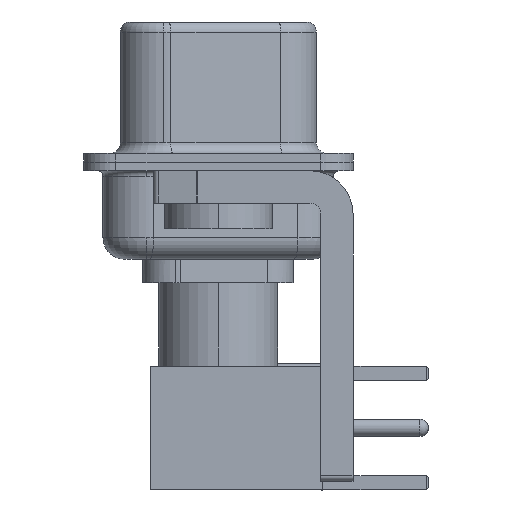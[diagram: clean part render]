
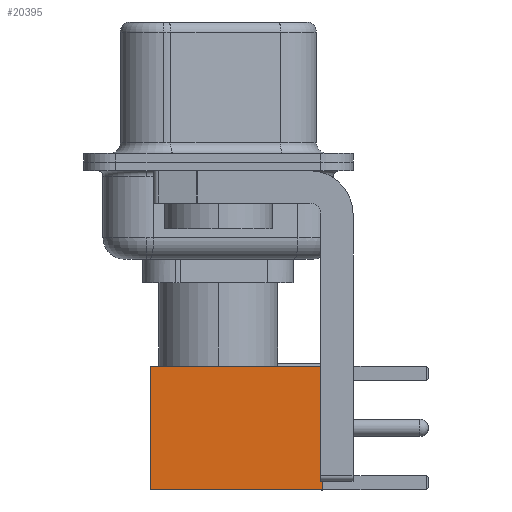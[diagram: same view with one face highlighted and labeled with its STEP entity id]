
A CAD part, left-side view. The second image highlights one B-rep face of the part: STEP entity #20395.
In plain terms, the highlighted face is planar.
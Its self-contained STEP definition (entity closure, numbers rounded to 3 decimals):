
#57 = EDGE_LOOP ( 'NONE', ( #11467, #21428, #1774, #12795 ) ) ;
#1203 = DIRECTION ( 'NONE',  ( 0., 0., -1. ) ) ;
#1774 = ORIENTED_EDGE ( 'NONE', *, *, #12895, .F. ) ;
#1850 = DIRECTION ( 'NONE',  ( 0., 0., 1. ) ) ;
#2025 = CARTESIAN_POINT ( 'NONE',  ( 2.875, 2.875, 0. ) ) ;
#4457 = EDGE_CURVE ( 'NONE', #24757, #23420, #13346, .T. ) ;
#4635 = VECTOR ( 'NONE', #1203, 1000. ) ;
#8365 = VERTEX_POINT ( 'NONE', #29465 ) ;
#8676 = VECTOR ( 'NONE', #19637, 1000. ) ;
#9818 = LINE ( 'NONE', #29973, #8676 ) ;
#9927 = CARTESIAN_POINT ( 'NONE',  ( -2.875, 2.875, 8. ) ) ;
#11467 = ORIENTED_EDGE ( 'NONE', *, *, #4457, .T. ) ;
#12017 = VECTOR ( 'NONE', #21219, 1000. ) ;
#12795 = ORIENTED_EDGE ( 'NONE', *, *, #19138, .F. ) ;
#12895 = EDGE_CURVE ( 'NONE', #24874, #8365, #24387, .T. ) ;
#13346 = LINE ( 'NONE', #18438, #33176 ) ;
#13581 = CARTESIAN_POINT ( 'NONE',  ( 0., 2.875, 0. ) ) ;
#18438 = CARTESIAN_POINT ( 'NONE',  ( 2.875, 2.875, 0. ) ) ;
#19138 = EDGE_CURVE ( 'NONE', #24757, #24874, #9818, .T. ) ;
#19474 = DIRECTION ( 'NONE',  ( 0., 1., 0. ) ) ;
#19637 = DIRECTION ( 'NONE',  ( -1., 0., 0. ) ) ;
#19932 = CARTESIAN_POINT ( 'NONE',  ( 2.875, 2.875, 8. ) ) ;
#20395 = ADVANCED_FACE ( 'NONE', ( #32514 ), #27433, .T. ) ;
#21219 = DIRECTION ( 'NONE',  ( -1., 0., 0. ) ) ;
#21428 = ORIENTED_EDGE ( 'NONE', *, *, #25558, .T. ) ;
#22179 = CARTESIAN_POINT ( 'NONE',  ( -2.875, 2.875, 0. ) ) ;
#22996 = CARTESIAN_POINT ( 'NONE',  ( 2.875, 2.875, 0. ) ) ;
#23420 = VERTEX_POINT ( 'NONE', #22996 ) ;
#24387 = LINE ( 'NONE', #22179, #4635 ) ;
#24757 = VERTEX_POINT ( 'NONE', #19932 ) ;
#24874 = VERTEX_POINT ( 'NONE', #9927 ) ;
#25558 = EDGE_CURVE ( 'NONE', #23420, #8365, #25954, .T. ) ;
#25954 = LINE ( 'NONE', #13581, #12017 ) ;
#27433 = PLANE ( 'NONE',  #32465 ) ;
#29465 = CARTESIAN_POINT ( 'NONE',  ( -2.875, 2.875, 0. ) ) ;
#29973 = CARTESIAN_POINT ( 'NONE',  ( 0., 2.875, 8. ) ) ;
#31313 = DIRECTION ( 'NONE',  ( 0., 0., -1. ) ) ;
#32465 = AXIS2_PLACEMENT_3D ( 'NONE', #2025, #19474, #1850 ) ;
#32514 = FACE_OUTER_BOUND ( 'NONE', #57, .T. ) ;
#33176 = VECTOR ( 'NONE', #31313, 1000. ) ;
